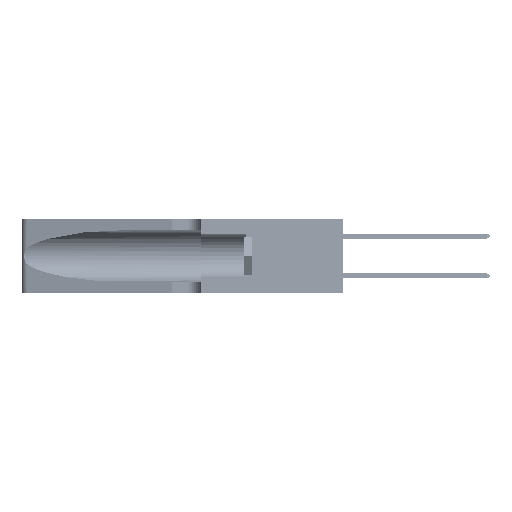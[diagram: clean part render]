
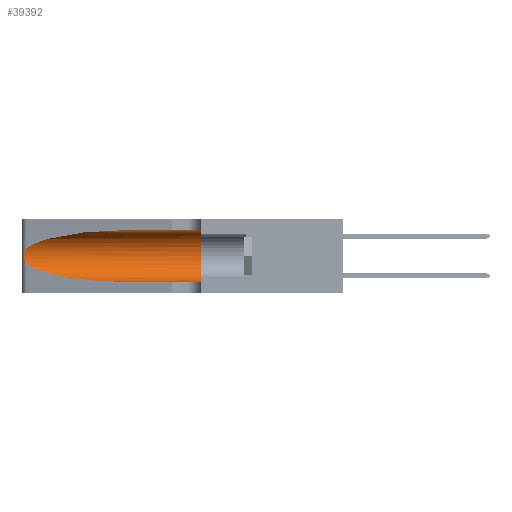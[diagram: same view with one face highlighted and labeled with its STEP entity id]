
A CAD part, left-side view. The second image highlights one B-rep face of the part: STEP entity #39392.
In plain terms, the highlighted cylindrical face has radius 3.308 mm (diameter 6.617 mm), a partial arc.
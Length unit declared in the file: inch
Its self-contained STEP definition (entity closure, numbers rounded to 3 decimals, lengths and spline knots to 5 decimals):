
#599 = VECTOR ( 'NONE', #17441, 39.37008 ) ;
#928 = ORIENTED_EDGE ( 'NONE', *, *, #28932, .T. ) ;
#1536 = CARTESIAN_POINT ( 'NONE',  ( 0.26018, 1.23835, 0.19895 ) ) ;
#2972 = CYLINDRICAL_SURFACE ( 'NONE', #42458, 0.13025 ) ;
#3563 = VERTEX_POINT ( 'NONE', #40381 ) ;
#3668 = CARTESIAN_POINT ( 'NONE',  ( 0.1305, 0.35, 0.185 ) ) ;
#3847 = DIRECTION ( 'NONE',  ( 0., 0., 1. ) ) ;
#5618 = CARTESIAN_POINT ( 'NONE',  ( 0.2373, 1.15595, 0.08982 ) ) ;
#5843 = CARTESIAN_POINT ( 'NONE',  ( 0.25787, 1.23484, 0.2124 ) ) ;
#6024 = CARTESIAN_POINT ( 'NONE',  ( 0.25487, 1.22718, 0.22369 ) ) ;
#6871 = VERTEX_POINT ( 'NONE', #35273 ) ;
#9468 = EDGE_LOOP ( 'NONE', ( #40850, #52440, #928, #13436, #23148, #34341 ) ) ;
#10651 = CARTESIAN_POINT ( 'NONE',  ( 0.1305, 1.61858, 0.185 ) ) ;
#13436 = ORIENTED_EDGE ( 'NONE', *, *, #37749, .T. ) ;
#13525 = CARTESIAN_POINT ( 'NONE',  ( 0.1305, 0.72297, 0.05475 ) ) ;
#13999 = DIRECTION ( 'NONE',  ( 0., -1., 0. ) ) ;
#14126 = CARTESIAN_POINT ( 'NONE',  ( 0.25854, 1.2359, 0.20912 ) ) ;
#15642 = CARTESIAN_POINT ( 'NONE',  ( 0.25487, 1.22718, 0.22369 ) ) ;
#17263 = EDGE_CURVE ( 'NONE', #44283, #21186, #52902, .T. ) ;
#17441 = DIRECTION ( 'NONE',  ( 0., -1., 0. ) ) ;
#18097 = CARTESIAN_POINT ( 'NONE',  ( 0.25789, 1.23486, 0.15765 ) ) ;
#18277 = CARTESIAN_POINT ( 'NONE',  ( 0.26075, 1.23896, 0.19203 ) ) ;
#21066 = CARTESIAN_POINT ( 'NONE',  ( 0.1305, 1.61858, 0.05475 ) ) ;
#21186 = VERTEX_POINT ( 'NONE', #15642 ) ;
#21862 = CARTESIAN_POINT ( 'NONE',  ( 0.25487, 1.22718, 0.14631 ) ) ;
#23148 = ORIENTED_EDGE ( 'NONE', *, *, #38951, .F. ) ;
#23422 = DIRECTION ( 'NONE',  ( 0., -1., 0. ) ) ;
#26386 = CARTESIAN_POINT ( 'NONE',  ( 0.25856, 1.23593, 0.16098 ) ) ;
#26864 = CARTESIAN_POINT ( 'NONE',  ( 0.25487, 1.22718, 0.22369 ) ) ;
#28628 = AXIS2_PLACEMENT_3D ( 'NONE', #3668, #49028, #3847 ) ;
#28932 = EDGE_CURVE ( 'NONE', #30846, #6871, #51282, .T. ) ;
#30141 = CARTESIAN_POINT ( 'NONE',  ( 0.25639, 1.23184, 0.21858 ) ) ;
#30358 = CARTESIAN_POINT ( 'NONE',  ( 0.1305, 1.61858, 0.31525 ) ) ;
#30749 = VERTEX_POINT ( 'NONE', #40439 ) ;
#30846 = VERTEX_POINT ( 'NONE', #21862 ) ;
#33385 = LINE ( 'NONE', #21066, #599 ) ;
#33747 = B_SPLINE_CURVE_WITH_KNOTS ( 'NONE', 3,
 ( #6024, #38757, #30141, #5843, #14126, #1536, #18277, #47069, #38582, #26386, #18097, #50669, #46893, #38949 ),
 .UNSPECIFIED., .F., .F.,
 ( 4, 2, 2, 2, 2, 2, 4 ),
 ( 0., 0.00027, 0.00053, 0.00107, 0.0016, 0.00187, 0.00214 ),
 .UNSPECIFIED. ) ;
#34018 = CARTESIAN_POINT ( 'NONE',  ( 0.18966, 0.96281, 0.31525 ) ) ;
#34341 = ORIENTED_EDGE ( 'NONE', *, *, #42517, .F. ) ;
#35273 = CARTESIAN_POINT ( 'NONE',  ( 0.1305, 0.72297, 0.05475 ) ) ;
#35300 = EDGE_CURVE ( 'NONE', #21186, #30846, #33747, .T. ) ;
#35474 = CARTESIAN_POINT ( 'NONE',  ( 0.2373, 1.15595, 0.28018 ) ) ;
#35993 = DIRECTION ( 'NONE',  ( 0., 0., -1. ) ) ;
#36936 = CARTESIAN_POINT ( 'NONE',  ( 0.1305, 0.72297, 0.31525 ) ) ;
#37749 = EDGE_CURVE ( 'NONE', #6871, #3563, #33385, .T. ) ;
#38582 = CARTESIAN_POINT ( 'NONE',  ( 0.26017, 1.23833, 0.17102 ) ) ;
#38757 = CARTESIAN_POINT ( 'NONE',  ( 0.25555, 1.22994, 0.2215 ) ) ;
#38949 = CARTESIAN_POINT ( 'NONE',  ( 0.25487, 1.22718, 0.14631 ) ) ;
#38951 = EDGE_CURVE ( 'NONE', #30749, #3563, #47443, .T. ) ;
#39078 = CARTESIAN_POINT ( 'NONE',  ( 0.1305, 0.72297, 0.31525 ) ) ;
#39392 = ADVANCED_FACE ( 'NONE', ( #48081 ), #2972, .F. ) ;
#40381 = CARTESIAN_POINT ( 'NONE',  ( 0.1305, 0.35, 0.05475 ) ) ;
#40439 = CARTESIAN_POINT ( 'NONE',  ( 0.1305, 0.35, 0.31525 ) ) ;
#40850 = ORIENTED_EDGE ( 'NONE', *, *, #17263, .T. ) ;
#42458 = AXIS2_PLACEMENT_3D ( 'NONE', #10651, #23422, #35993 ) ;
#42517 = EDGE_CURVE ( 'NONE', #44283, #30749, #49009, .T. ) ;
#42711 = CARTESIAN_POINT ( 'NONE',  ( 0.18966, 0.96281, 0.05475 ) ) ;
#44283 = VERTEX_POINT ( 'NONE', #36936 ) ;
#46893 = CARTESIAN_POINT ( 'NONE',  ( 0.25555, 1.22993, 0.14849 ) ) ;
#47069 = CARTESIAN_POINT ( 'NONE',  ( 0.26075, 1.23896, 0.178 ) ) ;
#47443 = CIRCLE ( 'NONE', #28628, 0.13025 ) ;
#48081 = FACE_OUTER_BOUND ( 'NONE', #9468, .T. ) ;
#49009 = LINE ( 'NONE', #30358, #50309 ) ;
#49028 = DIRECTION ( 'NONE',  ( 0., 1., 0. ) ) ;
#50309 = VECTOR ( 'NONE', #13999, 39.37008 ) ;
#50669 = CARTESIAN_POINT ( 'NONE',  ( 0.25639, 1.23186, 0.15144 ) ) ;
#50784 = CARTESIAN_POINT ( 'NONE',  ( 0.25487, 1.22718, 0.14631 ) ) ;
#51282 =( BOUNDED_CURVE ( )  B_SPLINE_CURVE ( 3, ( #50784, #5618, #42711, #13525 ),
 .UNSPECIFIED., .F., .F. ) 
 B_SPLINE_CURVE_WITH_KNOTS ( ( 4, 4 ),
 ( 3.44316, 4.71239 ),
 .UNSPECIFIED. ) 
 CURVE ( )  GEOMETRIC_REPRESENTATION_ITEM ( )  RATIONAL_B_SPLINE_CURVE ( ( 1., 0.87, 0.87, 1. ) ) 
 REPRESENTATION_ITEM ( '' )  );
#52440 = ORIENTED_EDGE ( 'NONE', *, *, #35300, .T. ) ;
#52902 =( BOUNDED_CURVE ( )  B_SPLINE_CURVE ( 3, ( #39078, #34018, #35474, #26864 ),
 .UNSPECIFIED., .F., .F. ) 
 B_SPLINE_CURVE_WITH_KNOTS ( ( 4, 4 ),
 ( 1.5708, 2.84003 ),
 .UNSPECIFIED. ) 
 CURVE ( )  GEOMETRIC_REPRESENTATION_ITEM ( )  RATIONAL_B_SPLINE_CURVE ( ( 1., 0.87, 0.87, 1. ) ) 
 REPRESENTATION_ITEM ( '' )  );
